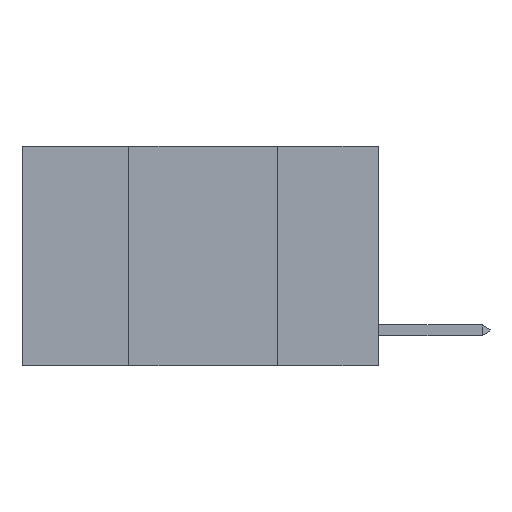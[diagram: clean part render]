
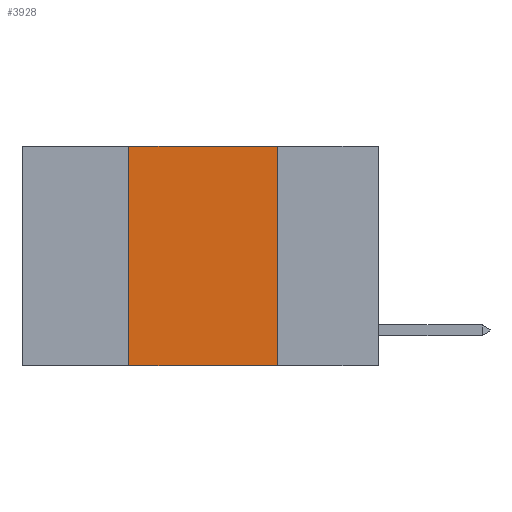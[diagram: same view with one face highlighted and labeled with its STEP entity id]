
A CAD part, left-side view. The second image highlights one B-rep face of the part: STEP entity #3928.
In plain terms, the highlighted planar face has unit normal (-1, 0, 0).
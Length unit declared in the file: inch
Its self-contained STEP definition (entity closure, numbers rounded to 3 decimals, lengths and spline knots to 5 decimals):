
#1572 = DIRECTION ( 'NONE',  ( 0., 0., -1. ) ) ;
#2102 = CARTESIAN_POINT ( 'NONE',  ( 0., 0.42, 0. ) ) ;
#2373 = VECTOR ( 'NONE', #1572, 39.37008 ) ;
#2663 = VERTEX_POINT ( 'NONE', #11971 ) ;
#2980 = CARTESIAN_POINT ( 'NONE',  ( 0., 0.42, 0. ) ) ;
#3148 = ORIENTED_EDGE ( 'NONE', *, *, #7404, .F. ) ;
#3891 = PLANE ( 'NONE',  #22516 ) ;
#3928 = ADVANCED_FACE ( 'NONE', ( #8035 ), #3891, .F. ) ;
#4175 = DIRECTION ( 'NONE',  ( 0., 0., 1. ) ) ;
#4646 = CARTESIAN_POINT ( 'NONE',  ( 0., 0.17, -0.37 ) ) ;
#4842 = VERTEX_POINT ( 'NONE', #4646 ) ;
#4964 = DIRECTION ( 'NONE',  ( 0., -1., 0. ) ) ;
#5752 = CARTESIAN_POINT ( 'NONE',  ( 0., 0.42, -0.37 ) ) ;
#7404 = EDGE_CURVE ( 'NONE', #25680, #2663, #15463, .T. ) ;
#7934 = ORIENTED_EDGE ( 'NONE', *, *, #21468, .F. ) ;
#7989 = CARTESIAN_POINT ( 'NONE',  ( 0., 0.6, 0. ) ) ;
#8035 = FACE_OUTER_BOUND ( 'NONE', #19292, .T. ) ;
#8523 = LINE ( 'NONE', #2102, #18579 ) ;
#10026 = DIRECTION ( 'NONE',  ( 0., 0., -1. ) ) ;
#11971 = CARTESIAN_POINT ( 'NONE',  ( 0., 0.17, 0. ) ) ;
#12860 = CARTESIAN_POINT ( 'NONE',  ( 0., 0.6, -0.37 ) ) ;
#13338 = VECTOR ( 'NONE', #4964, 39.37008 ) ;
#14796 = VERTEX_POINT ( 'NONE', #5752 ) ;
#15463 = LINE ( 'NONE', #15929, #19517 ) ;
#15880 = ORIENTED_EDGE ( 'NONE', *, *, #17506, .T. ) ;
#15929 = CARTESIAN_POINT ( 'NONE',  ( 0., 0.6, 0. ) ) ;
#17506 = EDGE_CURVE ( 'NONE', #14796, #4842, #18629, .T. ) ;
#17940 = DIRECTION ( 'NONE',  ( 0., -1., 0. ) ) ;
#18514 = LINE ( 'NONE', #25638, #2373 ) ;
#18579 = VECTOR ( 'NONE', #4175, 39.37008 ) ;
#18629 = LINE ( 'NONE', #12860, #13338 ) ;
#18834 = EDGE_CURVE ( 'NONE', #14796, #25680, #8523, .T. ) ;
#19292 = EDGE_LOOP ( 'NONE', ( #7934, #3148, #24090, #15880 ) ) ;
#19517 = VECTOR ( 'NONE', #17940, 39.37008 ) ;
#21468 = EDGE_CURVE ( 'NONE', #2663, #4842, #18514, .T. ) ;
#21977 = DIRECTION ( 'NONE',  ( 1., 0., 0. ) ) ;
#22516 = AXIS2_PLACEMENT_3D ( 'NONE', #7989, #21977, #10026 ) ;
#24090 = ORIENTED_EDGE ( 'NONE', *, *, #18834, .F. ) ;
#25638 = CARTESIAN_POINT ( 'NONE',  ( 0., 0.17, 0. ) ) ;
#25680 = VERTEX_POINT ( 'NONE', #2980 ) ;
